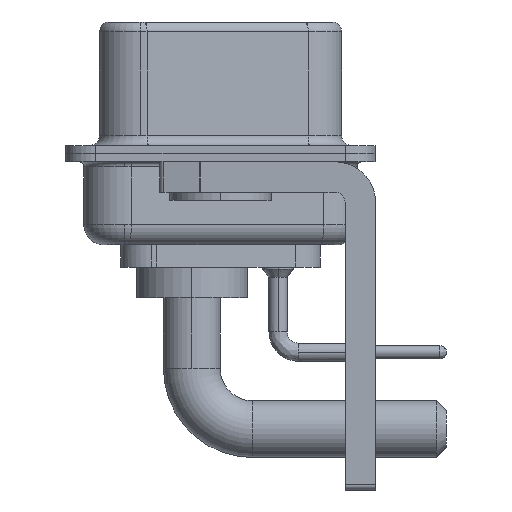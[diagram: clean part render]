
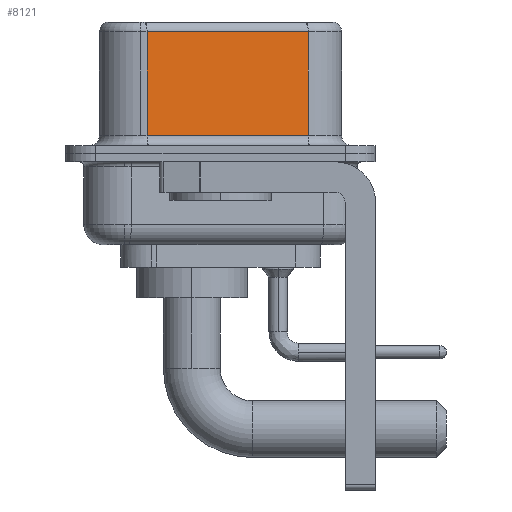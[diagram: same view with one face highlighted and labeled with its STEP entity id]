
A CAD part, left-side view. The second image highlights one B-rep face of the part: STEP entity #8121.
In plain terms, the highlighted planar face has unit normal (-0.985, -0.174, 0).
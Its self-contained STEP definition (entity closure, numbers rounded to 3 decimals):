
#850 = LINE ( 'NONE', #10561, #10064 ) ;
#993 = EDGE_LOOP ( 'NONE', ( #6263, #17812, #14348, #5632 ) ) ;
#1859 = LINE ( 'NONE', #16595, #7720 ) ;
#2838 = DIRECTION ( 'NONE',  ( 0., 0., -1. ) ) ;
#2980 = EDGE_CURVE ( 'NONE', #21317, #15773, #4960, .T. ) ;
#4410 = VERTEX_POINT ( 'NONE', #21262 ) ;
#4960 = LINE ( 'NONE', #18321, #12295 ) ;
#5582 = EDGE_CURVE ( 'NONE', #15773, #23753, #1859, .T. ) ;
#5632 = ORIENTED_EDGE ( 'NONE', *, *, #5582, .T. ) ;
#5963 = DIRECTION ( 'NONE',  ( 0.985, 0.174, 0. ) ) ;
#6263 = ORIENTED_EDGE ( 'NONE', *, *, #11741, .F. ) ;
#7720 = VECTOR ( 'NONE', #20818, 1000. ) ;
#8121 = ADVANCED_FACE ( 'NONE', ( #15341 ), #13466, .F. ) ;
#10064 = VECTOR ( 'NONE', #19686, 1000. ) ;
#10561 = CARTESIAN_POINT ( 'NONE',  ( 5.132, -4.322, 6.02 ) ) ;
#11741 = EDGE_CURVE ( 'NONE', #4410, #23753, #21659, .T. ) ;
#12295 = VECTOR ( 'NONE', #2838, 1000. ) ;
#12309 = CARTESIAN_POINT ( 'NONE',  ( 5.132, -4.322, 0.9 ) ) ;
#13466 = PLANE ( 'NONE',  #23979 ) ;
#13582 = DIRECTION ( 'NONE',  ( -0.174, 0.985, 0. ) ) ;
#14152 = VECTOR ( 'NONE', #16068, 1000. ) ;
#14156 = CARTESIAN_POINT ( 'NONE',  ( 3.73, 3.628, 0.9 ) ) ;
#14348 = ORIENTED_EDGE ( 'NONE', *, *, #2980, .T. ) ;
#15341 = FACE_OUTER_BOUND ( 'NONE', #993, .T. ) ;
#15773 = VERTEX_POINT ( 'NONE', #14156 ) ;
#15940 = CARTESIAN_POINT ( 'NONE',  ( 5.132, -4.322, 6.52 ) ) ;
#16068 = DIRECTION ( 'NONE',  ( 0., 0., -1. ) ) ;
#16595 = CARTESIAN_POINT ( 'NONE',  ( 5.132, -4.322, 0.9 ) ) ;
#17343 = CARTESIAN_POINT ( 'NONE',  ( 5.132, -4.322, 6.52 ) ) ;
#17812 = ORIENTED_EDGE ( 'NONE', *, *, #21134, .T. ) ;
#18321 = CARTESIAN_POINT ( 'NONE',  ( 3.73, 3.628, 6.52 ) ) ;
#19686 = DIRECTION ( 'NONE',  ( -0.174, 0.985, 0. ) ) ;
#20818 = DIRECTION ( 'NONE',  ( 0.174, -0.985, 0. ) ) ;
#21134 = EDGE_CURVE ( 'NONE', #4410, #21317, #850, .T. ) ;
#21262 = CARTESIAN_POINT ( 'NONE',  ( 5.132, -4.322, 6.02 ) ) ;
#21317 = VERTEX_POINT ( 'NONE', #24292 ) ;
#21659 = LINE ( 'NONE', #15940, #14152 ) ;
#23753 = VERTEX_POINT ( 'NONE', #12309 ) ;
#23979 = AXIS2_PLACEMENT_3D ( 'NONE', #17343, #5963, #13582 ) ;
#24292 = CARTESIAN_POINT ( 'NONE',  ( 3.73, 3.628, 6.02 ) ) ;
